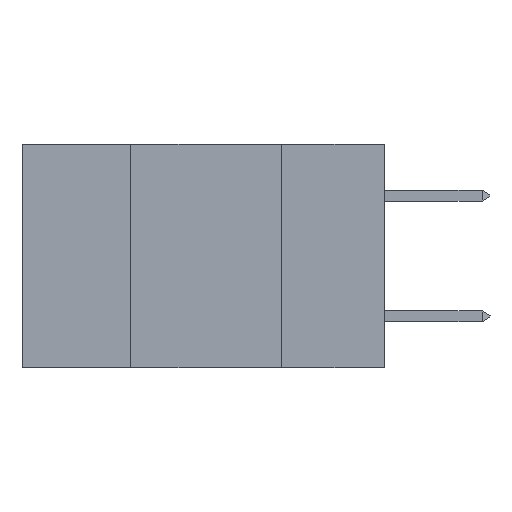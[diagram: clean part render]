
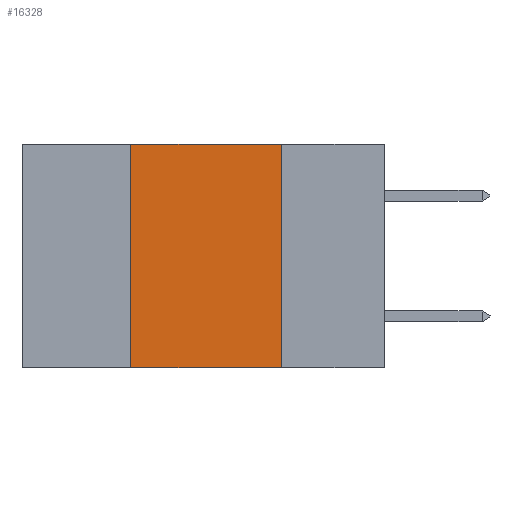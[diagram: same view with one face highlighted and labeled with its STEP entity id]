
A CAD part, left-side view. The second image highlights one B-rep face of the part: STEP entity #16328.
In plain terms, the highlighted planar face has unit normal (-1, 0, 0).
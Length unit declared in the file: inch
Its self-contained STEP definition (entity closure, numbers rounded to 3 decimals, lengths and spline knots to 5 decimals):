
#661 = VECTOR ( 'NONE', #7343, 39.37008 ) ;
#1200 = DIRECTION ( 'NONE',  ( 1., 0., 0. ) ) ;
#1372 = LINE ( 'NONE', #32097, #11621 ) ;
#3131 = EDGE_CURVE ( 'NONE', #20742, #16525, #1372, .T. ) ;
#3497 = LINE ( 'NONE', #13691, #4419 ) ;
#4419 = VECTOR ( 'NONE', #31889, 39.37008 ) ;
#4523 = ORIENTED_EDGE ( 'NONE', *, *, #30437, .F. ) ;
#5842 = EDGE_CURVE ( 'NONE', #27366, #17176, #17891, .T. ) ;
#6071 = CARTESIAN_POINT ( 'NONE',  ( 0., 0.42, 0. ) ) ;
#6554 = DIRECTION ( 'NONE',  ( 0., 0., 1. ) ) ;
#7343 = DIRECTION ( 'NONE',  ( 0., -1., 0. ) ) ;
#7718 = ORIENTED_EDGE ( 'NONE', *, *, #5842, .T. ) ;
#9355 = PLANE ( 'NONE',  #27857 ) ;
#10993 = EDGE_LOOP ( 'NONE', ( #30500, #30037, #4523, #7718 ) ) ;
#11258 = CARTESIAN_POINT ( 'NONE',  ( 0., 0.42, -0.37 ) ) ;
#11621 = VECTOR ( 'NONE', #21593, 39.37008 ) ;
#11818 = CARTESIAN_POINT ( 'NONE',  ( 0., 0.42, 0. ) ) ;
#13044 = CARTESIAN_POINT ( 'NONE',  ( 0., 0.6, -0.37 ) ) ;
#13691 = CARTESIAN_POINT ( 'NONE',  ( 0., 0.17, 0. ) ) ;
#16328 = ADVANCED_FACE ( 'NONE', ( #21904 ), #9355, .F. ) ;
#16525 = VERTEX_POINT ( 'NONE', #18067 ) ;
#17176 = VERTEX_POINT ( 'NONE', #29509 ) ;
#17891 = LINE ( 'NONE', #13044, #661 ) ;
#18067 = CARTESIAN_POINT ( 'NONE',  ( 0., 0.17, 0. ) ) ;
#20742 = VERTEX_POINT ( 'NONE', #11818 ) ;
#21593 = DIRECTION ( 'NONE',  ( 0., -1., 0. ) ) ;
#21904 = FACE_OUTER_BOUND ( 'NONE', #10993, .T. ) ;
#21934 = LINE ( 'NONE', #6071, #25340 ) ;
#24568 = DIRECTION ( 'NONE',  ( 0., 0., -1. ) ) ;
#25340 = VECTOR ( 'NONE', #6554, 39.37008 ) ;
#26432 = EDGE_CURVE ( 'NONE', #16525, #17176, #3497, .T. ) ;
#27366 = VERTEX_POINT ( 'NONE', #11258 ) ;
#27857 = AXIS2_PLACEMENT_3D ( 'NONE', #32264, #1200, #24568 ) ;
#29509 = CARTESIAN_POINT ( 'NONE',  ( 0., 0.17, -0.37 ) ) ;
#30037 = ORIENTED_EDGE ( 'NONE', *, *, #3131, .F. ) ;
#30437 = EDGE_CURVE ( 'NONE', #27366, #20742, #21934, .T. ) ;
#30500 = ORIENTED_EDGE ( 'NONE', *, *, #26432, .F. ) ;
#31889 = DIRECTION ( 'NONE',  ( 0., 0., -1. ) ) ;
#32097 = CARTESIAN_POINT ( 'NONE',  ( 0., 0.6, 0. ) ) ;
#32264 = CARTESIAN_POINT ( 'NONE',  ( 0., 0.6, 0. ) ) ;
